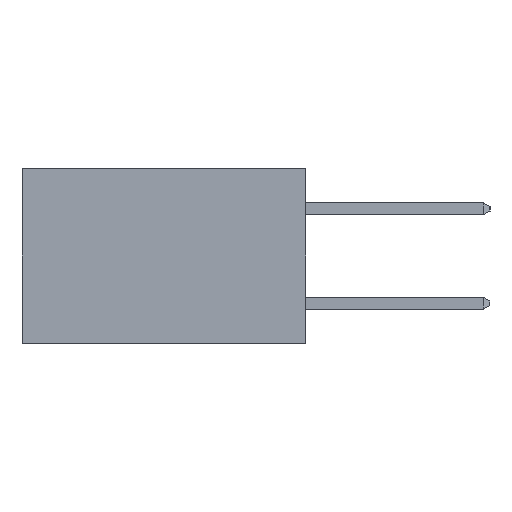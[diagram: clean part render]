
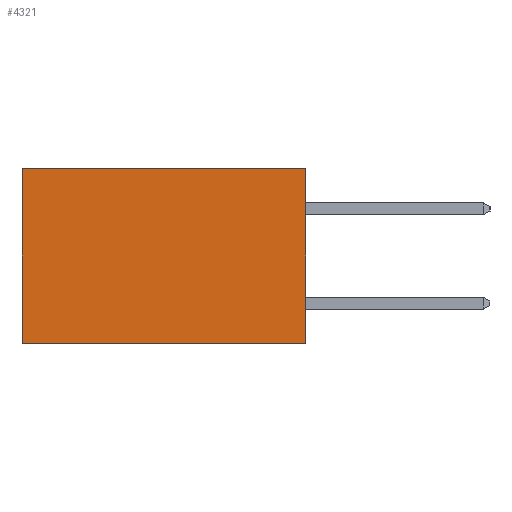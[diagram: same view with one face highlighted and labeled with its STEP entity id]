
A CAD part, left-side view. The second image highlights one B-rep face of the part: STEP entity #4321.
In plain terms, the highlighted planar face has unit normal (-1, 0, 0).
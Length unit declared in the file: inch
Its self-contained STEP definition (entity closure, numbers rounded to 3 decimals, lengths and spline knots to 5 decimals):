
#539 = CARTESIAN_POINT ( 'NONE',  ( 0.298, 0., 0. ) ) ;
#1017 = LINE ( 'NONE', #21619, #13584 ) ;
#1725 = LINE ( 'NONE', #7363, #12113 ) ;
#2050 = PLANE ( 'NONE',  #9031 ) ;
#2575 = ORIENTED_EDGE ( 'NONE', *, *, #4107, .T. ) ;
#2599 = VECTOR ( 'NONE', #8112, 39.37008 ) ;
#4107 = EDGE_CURVE ( 'NONE', #14067, #20293, #1017, .T. ) ;
#4321 = ADVANCED_FACE ( 'NONE', ( #19017 ), #2050, .F. ) ;
#4784 = DIRECTION ( 'NONE',  ( 0., 0., -1. ) ) ;
#4857 = DIRECTION ( 'NONE',  ( 1., 0., 0. ) ) ;
#5335 = CARTESIAN_POINT ( 'NONE',  ( 0.298, 0.6, -0.37 ) ) ;
#5893 = CARTESIAN_POINT ( 'NONE',  ( 0.298, 0., -0.37 ) ) ;
#6457 = CARTESIAN_POINT ( 'NONE',  ( 0.298, 0., 0. ) ) ;
#6976 = ORIENTED_EDGE ( 'NONE', *, *, #17322, .T. ) ;
#7363 = CARTESIAN_POINT ( 'NONE',  ( 0.298, 0.6, 0. ) ) ;
#7861 = LINE ( 'NONE', #26039, #18822 ) ;
#8112 = DIRECTION ( 'NONE',  ( 0., 1., 0. ) ) ;
#8672 = DIRECTION ( 'NONE',  ( 0., 0., -1. ) ) ;
#9031 = AXIS2_PLACEMENT_3D ( 'NONE', #539, #4857, #4784 ) ;
#12113 = VECTOR ( 'NONE', #20490, 39.37008 ) ;
#13584 = VECTOR ( 'NONE', #16108, 39.37008 ) ;
#14067 = VERTEX_POINT ( 'NONE', #6457 ) ;
#15122 = VERTEX_POINT ( 'NONE', #5335 ) ;
#16108 = DIRECTION ( 'NONE',  ( 0., 1., 0. ) ) ;
#16938 = EDGE_LOOP ( 'NONE', ( #6976, #24559, #23329, #2575 ) ) ;
#17322 = EDGE_CURVE ( 'NONE', #20293, #15122, #1725, .T. ) ;
#18822 = VECTOR ( 'NONE', #8672, 39.37008 ) ;
#19017 = FACE_OUTER_BOUND ( 'NONE', #16938, .T. ) ;
#20144 = LINE ( 'NONE', #5893, #2599 ) ;
#20293 = VERTEX_POINT ( 'NONE', #21542 ) ;
#20490 = DIRECTION ( 'NONE',  ( 0., 0., -1. ) ) ;
#20760 = EDGE_CURVE ( 'NONE', #25899, #15122, #20144, .T. ) ;
#21542 = CARTESIAN_POINT ( 'NONE',  ( 0.298, 0.6, 0. ) ) ;
#21619 = CARTESIAN_POINT ( 'NONE',  ( 0.298, 0., 0. ) ) ;
#23329 = ORIENTED_EDGE ( 'NONE', *, *, #25090, .F. ) ;
#24559 = ORIENTED_EDGE ( 'NONE', *, *, #20760, .F. ) ;
#25090 = EDGE_CURVE ( 'NONE', #14067, #25899, #7861, .T. ) ;
#25899 = VERTEX_POINT ( 'NONE', #26551 ) ;
#26039 = CARTESIAN_POINT ( 'NONE',  ( 0.298, 0., 0. ) ) ;
#26551 = CARTESIAN_POINT ( 'NONE',  ( 0.298, 0., -0.37 ) ) ;
